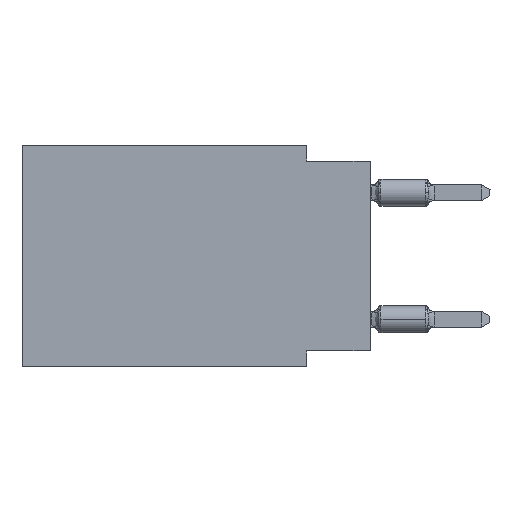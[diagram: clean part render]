
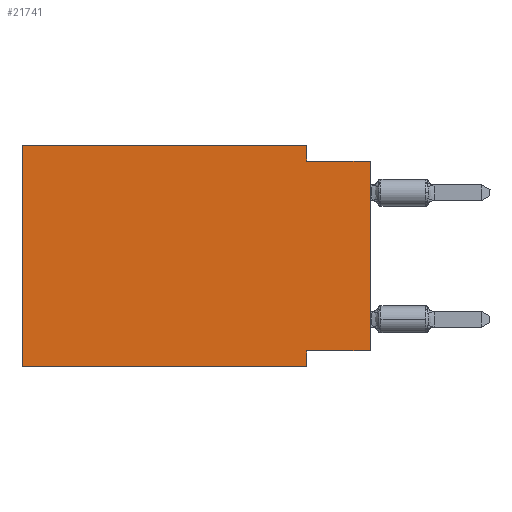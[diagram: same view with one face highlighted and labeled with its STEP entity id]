
A CAD part, left-side view. The second image highlights one B-rep face of the part: STEP entity #21741.
In plain terms, the highlighted planar face has unit normal (-1, 0, 0).
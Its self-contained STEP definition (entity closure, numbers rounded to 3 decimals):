
#255 = VECTOR ( 'NONE', #14134, 1000. ) ;
#1057 = ORIENTED_EDGE ( 'NONE', *, *, #22310, .F. ) ;
#2044 = LINE ( 'NONE', #11890, #255 ) ;
#2739 = CARTESIAN_POINT ( 'NONE',  ( 0., 0., -8.255 ) ) ;
#2929 = ORIENTED_EDGE ( 'NONE', *, *, #21781, .F. ) ;
#3374 = ORIENTED_EDGE ( 'NONE', *, *, #17639, .F. ) ;
#3776 = CARTESIAN_POINT ( 'NONE',  ( 0., 2.54, -8.89 ) ) ;
#4229 = EDGE_LOOP ( 'NONE', ( #8601, #16648, #23727, #2929, #10464, #16406, #3374, #1057 ) ) ;
#4247 = DIRECTION ( 'NONE',  ( 0., 0., -1. ) ) ;
#4770 = DIRECTION ( 'NONE',  ( 0., -1., 0. ) ) ;
#4961 = VECTOR ( 'NONE', #19448, 1000. ) ;
#6025 = CARTESIAN_POINT ( 'NONE',  ( 0., 0., -8.255 ) ) ;
#6037 = CARTESIAN_POINT ( 'NONE',  ( 0., 2.54, -8.255 ) ) ;
#6238 = CARTESIAN_POINT ( 'NONE',  ( 0., 2.54, -8.89 ) ) ;
#6829 = LINE ( 'NONE', #18879, #13747 ) ;
#7218 = VECTOR ( 'NONE', #16565, 1000. ) ;
#8251 = DIRECTION ( 'NONE',  ( 1., 0., 0. ) ) ;
#8353 = CARTESIAN_POINT ( 'NONE',  ( 0., 2.54, 0. ) ) ;
#8491 = LINE ( 'NONE', #8353, #7218 ) ;
#8601 = ORIENTED_EDGE ( 'NONE', *, *, #25570, .T. ) ;
#9510 = CARTESIAN_POINT ( 'NONE',  ( 0., 0., -0.635 ) ) ;
#9967 = EDGE_CURVE ( 'NONE', #23352, #12650, #21635, .T. ) ;
#10014 = AXIS2_PLACEMENT_3D ( 'NONE', #18321, #8251, #10111 ) ;
#10111 = DIRECTION ( 'NONE',  ( 0., 0., -1. ) ) ;
#10411 = CARTESIAN_POINT ( 'NONE',  ( 0., 2.54, -0.635 ) ) ;
#10464 = ORIENTED_EDGE ( 'NONE', *, *, #21477, .F. ) ;
#10929 = CARTESIAN_POINT ( 'NONE',  ( 0., 13.97, 0. ) ) ;
#11890 = CARTESIAN_POINT ( 'NONE',  ( 0., 0., 0. ) ) ;
#12650 = VERTEX_POINT ( 'NONE', #3776 ) ;
#12833 = LINE ( 'NONE', #2739, #4961 ) ;
#12859 = VERTEX_POINT ( 'NONE', #10411 ) ;
#12866 = FACE_OUTER_BOUND ( 'NONE', #4229, .T. ) ;
#13747 = VECTOR ( 'NONE', #24995, 1000. ) ;
#13874 = VECTOR ( 'NONE', #21141, 1000. ) ;
#14134 = DIRECTION ( 'NONE',  ( 0., 0., 1. ) ) ;
#16406 = ORIENTED_EDGE ( 'NONE', *, *, #9967, .T. ) ;
#16565 = DIRECTION ( 'NONE',  ( 0., 0., -1. ) ) ;
#16648 = ORIENTED_EDGE ( 'NONE', *, *, #24467, .F. ) ;
#16953 = CARTESIAN_POINT ( 'NONE',  ( 0., 13.97, 0. ) ) ;
#17639 = EDGE_CURVE ( 'NONE', #24353, #12650, #24408, .T. ) ;
#18051 = CARTESIAN_POINT ( 'NONE',  ( 0., 13.97, 0. ) ) ;
#18127 = VECTOR ( 'NONE', #4247, 1000. ) ;
#18321 = CARTESIAN_POINT ( 'NONE',  ( 0., 13.97, 0. ) ) ;
#18486 = CARTESIAN_POINT ( 'NONE',  ( 0., 13.97, -8.89 ) ) ;
#18879 = CARTESIAN_POINT ( 'NONE',  ( 0., 0., -0.635 ) ) ;
#19003 = LINE ( 'NONE', #10929, #13874 ) ;
#19448 = DIRECTION ( 'NONE',  ( 0., 1., 0. ) ) ;
#19497 = VERTEX_POINT ( 'NONE', #16953 ) ;
#20469 = EDGE_CURVE ( 'NONE', #22303, #12859, #8491, .T. ) ;
#20826 = VECTOR ( 'NONE', #25996, 1000. ) ;
#21141 = DIRECTION ( 'NONE',  ( 0., 0., 1. ) ) ;
#21302 = VERTEX_POINT ( 'NONE', #6025 ) ;
#21477 = EDGE_CURVE ( 'NONE', #23352, #19497, #19003, .T. ) ;
#21635 = LINE ( 'NONE', #25614, #20826 ) ;
#21741 = ADVANCED_FACE ( 'NONE', ( #12866 ), #24923, .F. ) ;
#21781 = EDGE_CURVE ( 'NONE', #19497, #22303, #22936, .T. ) ;
#22284 = VECTOR ( 'NONE', #4770, 1000. ) ;
#22303 = VERTEX_POINT ( 'NONE', #25023 ) ;
#22310 = EDGE_CURVE ( 'NONE', #21302, #24353, #12833, .T. ) ;
#22378 = VERTEX_POINT ( 'NONE', #9510 ) ;
#22936 = LINE ( 'NONE', #18051, #22284 ) ;
#23352 = VERTEX_POINT ( 'NONE', #18486 ) ;
#23727 = ORIENTED_EDGE ( 'NONE', *, *, #20469, .F. ) ;
#24353 = VERTEX_POINT ( 'NONE', #6037 ) ;
#24408 = LINE ( 'NONE', #6238, #18127 ) ;
#24467 = EDGE_CURVE ( 'NONE', #12859, #22378, #6829, .T. ) ;
#24923 = PLANE ( 'NONE',  #10014 ) ;
#24995 = DIRECTION ( 'NONE',  ( 0., -1., 0. ) ) ;
#25023 = CARTESIAN_POINT ( 'NONE',  ( 0., 2.54, 0. ) ) ;
#25570 = EDGE_CURVE ( 'NONE', #21302, #22378, #2044, .T. ) ;
#25614 = CARTESIAN_POINT ( 'NONE',  ( 0., 13.97, -8.89 ) ) ;
#25996 = DIRECTION ( 'NONE',  ( 0., -1., 0. ) ) ;
